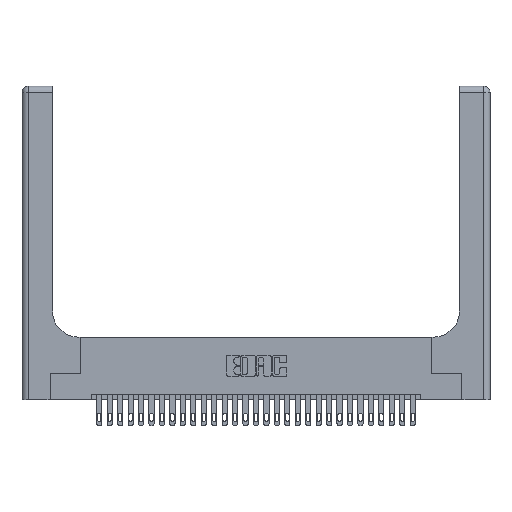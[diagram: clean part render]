
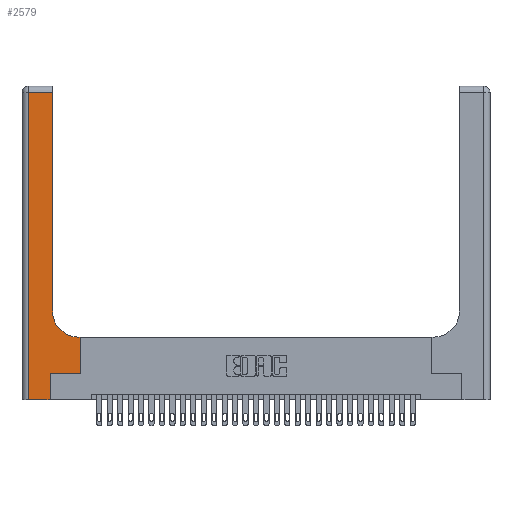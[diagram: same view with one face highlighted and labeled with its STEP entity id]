
A CAD part, top view. The second image highlights one B-rep face of the part: STEP entity #2579.
In plain terms, the highlighted planar face has unit normal (0, 0, 1).
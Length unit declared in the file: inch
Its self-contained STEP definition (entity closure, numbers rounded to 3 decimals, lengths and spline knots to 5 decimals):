
#169 = CARTESIAN_POINT ( 'NONE',  ( 0.2915, 3., 0.37 ) ) ;
#430 = CARTESIAN_POINT ( 'NONE',  ( 0.06, 0., 0.37 ) ) ;
#1501 = EDGE_CURVE ( 'NONE', #17720, #26144, #15149, .T. ) ;
#1674 = CARTESIAN_POINT ( 'NONE',  ( 0.2915, 0.6, 0.37 ) ) ;
#2579 = ADVANCED_FACE ( 'NONE', ( #23704 ), #14142, .F. ) ;
#2794 = CARTESIAN_POINT ( 'NONE',  ( 0.2915, 2.94, 0.37 ) ) ;
#3399 = DIRECTION ( 'NONE',  ( 1., 0., 0. ) ) ;
#4064 = LINE ( 'NONE', #18240, #11539 ) ;
#4232 = LINE ( 'NONE', #1674, #29206 ) ;
#4460 = EDGE_CURVE ( 'NONE', #19594, #22494, #4866, .T. ) ;
#4839 = CARTESIAN_POINT ( 'NONE',  ( 0.06, 2.94, 0.37 ) ) ;
#4866 = LINE ( 'NONE', #21698, #8629 ) ;
#4889 = ORIENTED_EDGE ( 'NONE', *, *, #18494, .T. ) ;
#5069 = DIRECTION ( 'NONE',  ( 1., 0., 0. ) ) ;
#6490 = AXIS2_PLACEMENT_3D ( 'NONE', #28519, #12039, #16543 ) ;
#6728 = LINE ( 'NONE', #21673, #25803 ) ;
#7794 = CARTESIAN_POINT ( 'NONE',  ( 0.5415, 0.85, 0.37 ) ) ;
#8629 = VECTOR ( 'NONE', #9790, 39.37008 ) ;
#9407 = CIRCLE ( 'NONE', #19891, 0.25 ) ;
#9790 = DIRECTION ( 'NONE',  ( 0., 1., 0. ) ) ;
#9905 = VERTEX_POINT ( 'NONE', #18520 ) ;
#10618 = DIRECTION ( 'NONE',  ( 0., 0., -1. ) ) ;
#10880 = ORIENTED_EDGE ( 'NONE', *, *, #14724, .T. ) ;
#10889 = LINE ( 'NONE', #18746, #23973 ) ;
#11178 = CARTESIAN_POINT ( 'NONE',  ( 0.269, 0., 0.37 ) ) ;
#11221 = ORIENTED_EDGE ( 'NONE', *, *, #4460, .T. ) ;
#11261 = VERTEX_POINT ( 'NONE', #14829 ) ;
#11298 = EDGE_CURVE ( 'NONE', #11261, #17720, #9407, .T. ) ;
#11539 = VECTOR ( 'NONE', #25153, 39.37008 ) ;
#12039 = DIRECTION ( 'NONE',  ( 0., 0., -1. ) ) ;
#13078 = VECTOR ( 'NONE', #14709, 39.37008 ) ;
#13809 = CARTESIAN_POINT ( 'NONE',  ( 0.5585, 0.25, 0.37 ) ) ;
#13846 = ORIENTED_EDGE ( 'NONE', *, *, #28231, .T. ) ;
#14065 = VERTEX_POINT ( 'NONE', #430 ) ;
#14142 = PLANE ( 'NONE',  #6490 ) ;
#14587 = ORIENTED_EDGE ( 'NONE', *, *, #16122, .T. ) ;
#14709 = DIRECTION ( 'NONE',  ( -1., 0., 0. ) ) ;
#14724 = EDGE_CURVE ( 'NONE', #14065, #29976, #6728, .T. ) ;
#14829 = CARTESIAN_POINT ( 'NONE',  ( 0.5415, 0.6, 0.37 ) ) ;
#15149 = LINE ( 'NONE', #169, #25970 ) ;
#16122 = EDGE_CURVE ( 'NONE', #29976, #9905, #4064, .T. ) ;
#16543 = DIRECTION ( 'NONE',  ( -1., 0., 0. ) ) ;
#16715 = ORIENTED_EDGE ( 'NONE', *, *, #19197, .T. ) ;
#17013 = CARTESIAN_POINT ( 'NONE',  ( 0., 2.94, 0.37 ) ) ;
#17720 = VERTEX_POINT ( 'NONE', #20803 ) ;
#18102 = ORIENTED_EDGE ( 'NONE', *, *, #26521, .T. ) ;
#18240 = CARTESIAN_POINT ( 'NONE',  ( 0.269, 0., 0.37 ) ) ;
#18494 = EDGE_CURVE ( 'NONE', #20389, #14065, #10889, .T. ) ;
#18520 = CARTESIAN_POINT ( 'NONE',  ( 0.269, 0.25, 0.37 ) ) ;
#18746 = CARTESIAN_POINT ( 'NONE',  ( 0.06, 3., 0.37 ) ) ;
#19197 = EDGE_CURVE ( 'NONE', #26144, #20389, #22443, .T. ) ;
#19212 = CARTESIAN_POINT ( 'NONE',  ( 0.269, 0.25, 0.37 ) ) ;
#19355 = DIRECTION ( 'NONE',  ( 0., 1., 0. ) ) ;
#19594 = VERTEX_POINT ( 'NONE', #13809 ) ;
#19891 = AXIS2_PLACEMENT_3D ( 'NONE', #7794, #10618, #3399 ) ;
#20389 = VERTEX_POINT ( 'NONE', #4839 ) ;
#20428 = DIRECTION ( 'NONE',  ( -1., 0., 0. ) ) ;
#20803 = CARTESIAN_POINT ( 'NONE',  ( 0.2915, 0.85, 0.37 ) ) ;
#21162 = EDGE_LOOP ( 'NONE', ( #26401, #16715, #4889, #10880, #14587, #18102, #11221, #13846, #26270 ) ) ;
#21673 = CARTESIAN_POINT ( 'NONE',  ( 0., 0., 0.37 ) ) ;
#21698 = CARTESIAN_POINT ( 'NONE',  ( 0.5585, 0.25, 0.37 ) ) ;
#22283 = VECTOR ( 'NONE', #5069, 39.37008 ) ;
#22443 = LINE ( 'NONE', #17013, #13078 ) ;
#22494 = VERTEX_POINT ( 'NONE', #27260 ) ;
#23704 = FACE_OUTER_BOUND ( 'NONE', #21162, .T. ) ;
#23973 = VECTOR ( 'NONE', #28419, 39.37008 ) ;
#24096 = DIRECTION ( 'NONE',  ( 1., 0., 0. ) ) ;
#24533 = LINE ( 'NONE', #19212, #22283 ) ;
#25153 = DIRECTION ( 'NONE',  ( 0., 1., 0. ) ) ;
#25803 = VECTOR ( 'NONE', #24096, 39.37008 ) ;
#25970 = VECTOR ( 'NONE', #19355, 39.37008 ) ;
#26144 = VERTEX_POINT ( 'NONE', #2794 ) ;
#26270 = ORIENTED_EDGE ( 'NONE', *, *, #11298, .T. ) ;
#26401 = ORIENTED_EDGE ( 'NONE', *, *, #1501, .T. ) ;
#26521 = EDGE_CURVE ( 'NONE', #9905, #19594, #24533, .T. ) ;
#27260 = CARTESIAN_POINT ( 'NONE',  ( 0.5585, 0.6, 0.37 ) ) ;
#28231 = EDGE_CURVE ( 'NONE', #22494, #11261, #4232, .T. ) ;
#28419 = DIRECTION ( 'NONE',  ( 0., -1., 0. ) ) ;
#28519 = CARTESIAN_POINT ( 'NONE',  ( 0., 3., 0.37 ) ) ;
#29206 = VECTOR ( 'NONE', #20428, 39.37008 ) ;
#29976 = VERTEX_POINT ( 'NONE', #11178 ) ;
